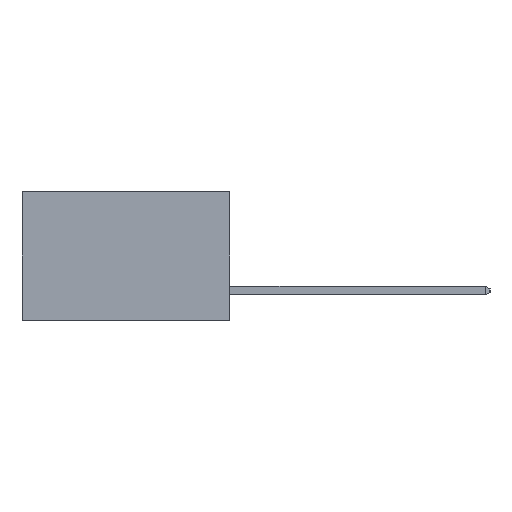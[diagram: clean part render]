
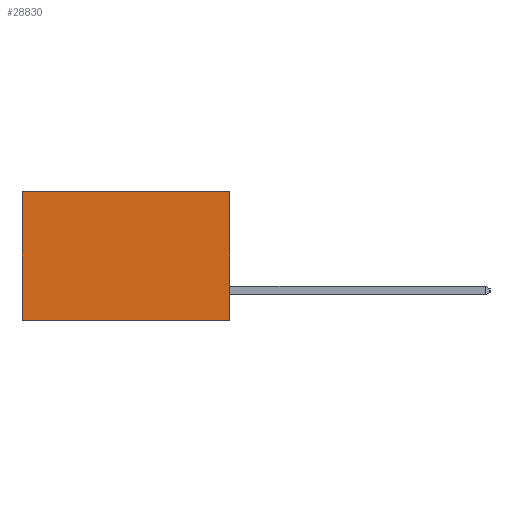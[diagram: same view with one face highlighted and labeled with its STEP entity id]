
A CAD part, left-side view. The second image highlights one B-rep face of the part: STEP entity #28830.
In plain terms, the highlighted planar face has unit normal (-1, 0, 0).
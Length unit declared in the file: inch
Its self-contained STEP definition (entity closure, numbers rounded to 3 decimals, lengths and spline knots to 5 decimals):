
#37 = VERTEX_POINT ( 'NONE', #28020 ) ;
#1472 = EDGE_CURVE ( 'NONE', #29843, #37, #2225, .T. ) ;
#2225 = LINE ( 'NONE', #12459, #26694 ) ;
#2757 = LINE ( 'NONE', #13984, #20936 ) ;
#4671 = EDGE_CURVE ( 'NONE', #11166, #16522, #2757, .T. ) ;
#4798 = DIRECTION ( 'NONE',  ( 0., 1., 0. ) ) ;
#6375 = AXIS2_PLACEMENT_3D ( 'NONE', #11103, #13653, #30108 ) ;
#10505 = VECTOR ( 'NONE', #4798, 39.37008 ) ;
#10637 = EDGE_LOOP ( 'NONE', ( #29544, #22640, #18997, #10876 ) ) ;
#10876 = ORIENTED_EDGE ( 'NONE', *, *, #15683, .T. ) ;
#10892 = CARTESIAN_POINT ( 'NONE',  ( 0.298, 0., -0.37 ) ) ;
#11103 = CARTESIAN_POINT ( 'NONE',  ( 0.298, 0., 0. ) ) ;
#11166 = VERTEX_POINT ( 'NONE', #26751 ) ;
#12316 = EDGE_CURVE ( 'NONE', #16522, #37, #16891, .T. ) ;
#12459 = CARTESIAN_POINT ( 'NONE',  ( 0.298, 0.6, 0. ) ) ;
#13531 = DIRECTION ( 'NONE',  ( 0., 0., -1. ) ) ;
#13653 = DIRECTION ( 'NONE',  ( 1., 0., 0. ) ) ;
#13984 = CARTESIAN_POINT ( 'NONE',  ( 0.298, 0., 0. ) ) ;
#14227 = CARTESIAN_POINT ( 'NONE',  ( 0.298, 0., -0.37 ) ) ;
#15403 = FACE_OUTER_BOUND ( 'NONE', #10637, .T. ) ;
#15683 = EDGE_CURVE ( 'NONE', #11166, #29843, #17810, .T. ) ;
#16522 = VERTEX_POINT ( 'NONE', #10892 ) ;
#16891 = LINE ( 'NONE', #14227, #10505 ) ;
#17810 = LINE ( 'NONE', #19891, #28795 ) ;
#18997 = ORIENTED_EDGE ( 'NONE', *, *, #4671, .F. ) ;
#19891 = CARTESIAN_POINT ( 'NONE',  ( 0.298, 0., 0. ) ) ;
#20936 = VECTOR ( 'NONE', #23367, 39.37008 ) ;
#22261 = DIRECTION ( 'NONE',  ( 0., 1., 0. ) ) ;
#22640 = ORIENTED_EDGE ( 'NONE', *, *, #12316, .F. ) ;
#23367 = DIRECTION ( 'NONE',  ( 0., 0., -1. ) ) ;
#26694 = VECTOR ( 'NONE', #13531, 39.37008 ) ;
#26751 = CARTESIAN_POINT ( 'NONE',  ( 0.298, 0., 0. ) ) ;
#27751 = PLANE ( 'NONE',  #6375 ) ;
#28020 = CARTESIAN_POINT ( 'NONE',  ( 0.298, 0.6, -0.37 ) ) ;
#28795 = VECTOR ( 'NONE', #22261, 39.37008 ) ;
#28826 = CARTESIAN_POINT ( 'NONE',  ( 0.298, 0.6, 0. ) ) ;
#28830 = ADVANCED_FACE ( 'NONE', ( #15403 ), #27751, .F. ) ;
#29544 = ORIENTED_EDGE ( 'NONE', *, *, #1472, .T. ) ;
#29843 = VERTEX_POINT ( 'NONE', #28826 ) ;
#30108 = DIRECTION ( 'NONE',  ( 0., 0., -1. ) ) ;
